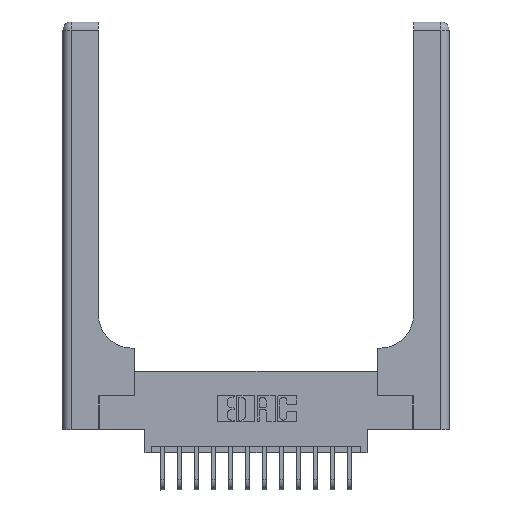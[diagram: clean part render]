
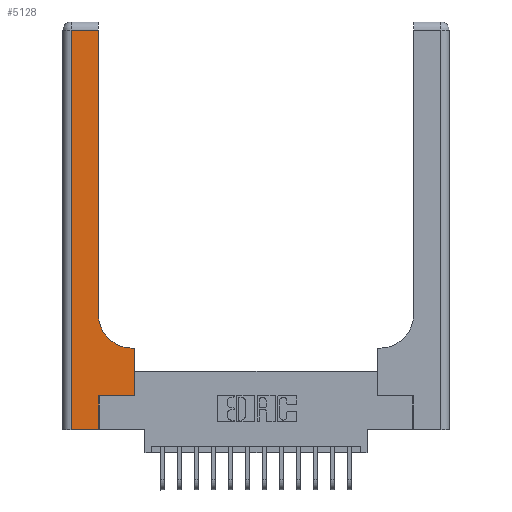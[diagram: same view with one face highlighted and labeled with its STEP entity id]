
A CAD part, top view. The second image highlights one B-rep face of the part: STEP entity #5128.
In plain terms, the highlighted planar face has unit normal (0, 0, 1).
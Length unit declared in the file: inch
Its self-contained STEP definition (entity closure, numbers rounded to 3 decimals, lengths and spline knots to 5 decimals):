
#183 = VERTEX_POINT ( 'NONE', #13406 ) ;
#333 = CARTESIAN_POINT ( 'NONE',  ( 0.06, 0., 0.37 ) ) ;
#395 = LINE ( 'NONE', #5743, #4962 ) ;
#425 = ORIENTED_EDGE ( 'NONE', *, *, #15638, .T. ) ;
#802 = VERTEX_POINT ( 'NONE', #10379 ) ;
#989 = ORIENTED_EDGE ( 'NONE', *, *, #3616, .T. ) ;
#1269 = EDGE_CURVE ( 'NONE', #12858, #1861, #12002, .T. ) ;
#1292 = DIRECTION ( 'NONE',  ( -1., 0., 0. ) ) ;
#1320 = DIRECTION ( 'NONE',  ( 1., 0., 0. ) ) ;
#1595 = LINE ( 'NONE', #17290, #9829 ) ;
#1654 = ORIENTED_EDGE ( 'NONE', *, *, #13908, .T. ) ;
#1861 = VERTEX_POINT ( 'NONE', #13651 ) ;
#2152 = VERTEX_POINT ( 'NONE', #13627 ) ;
#2262 = EDGE_CURVE ( 'NONE', #183, #13334, #3917, .T. ) ;
#2563 = EDGE_CURVE ( 'NONE', #5807, #802, #9725, .T. ) ;
#2675 = CARTESIAN_POINT ( 'NONE',  ( 0., 2.94, 0.37 ) ) ;
#2682 = CARTESIAN_POINT ( 'NONE',  ( 0.265, 0.25, 0.37 ) ) ;
#2789 = DIRECTION ( 'NONE',  ( -1., 0., 0. ) ) ;
#3233 = ORIENTED_EDGE ( 'NONE', *, *, #17201, .T. ) ;
#3318 = DIRECTION ( 'NONE',  ( 0., -1., 0. ) ) ;
#3373 = EDGE_CURVE ( 'NONE', #802, #12858, #7390, .T. ) ;
#3417 = CARTESIAN_POINT ( 'NONE',  ( 0.51, 0.85, 0.37 ) ) ;
#3509 = VERTEX_POINT ( 'NONE', #16862 ) ;
#3616 = EDGE_CURVE ( 'NONE', #1861, #3509, #1595, .T. ) ;
#3917 = CIRCLE ( 'NONE', #12902, 0.25 ) ;
#4319 = VECTOR ( 'NONE', #3318, 39.37008 ) ;
#4962 = VECTOR ( 'NONE', #12499, 39.37008 ) ;
#5128 = ADVANCED_FACE ( 'NONE', ( #17272 ), #9367, .F. ) ;
#5510 = CARTESIAN_POINT ( 'NONE',  ( 0.265, 0.25, 0.37 ) ) ;
#5743 = CARTESIAN_POINT ( 'NONE',  ( 0.26, 0.6, 0.37 ) ) ;
#5748 = ORIENTED_EDGE ( 'NONE', *, *, #7207, .T. ) ;
#5807 = VERTEX_POINT ( 'NONE', #333 ) ;
#6275 = VECTOR ( 'NONE', #13672, 39.37008 ) ;
#6960 = LINE ( 'NONE', #2675, #16210 ) ;
#7075 = CARTESIAN_POINT ( 'NONE',  ( 0.06, 3., 0.37 ) ) ;
#7207 = EDGE_CURVE ( 'NONE', #13334, #12428, #16456, .T. ) ;
#7390 = LINE ( 'NONE', #15204, #15443 ) ;
#7636 = DIRECTION ( 'NONE',  ( 0., 0., -1. ) ) ;
#8068 = ORIENTED_EDGE ( 'NONE', *, *, #1269, .T. ) ;
#8436 = CARTESIAN_POINT ( 'NONE',  ( 0.26, 0.85, 0.37 ) ) ;
#8875 = DIRECTION ( 'NONE',  ( 1., 0., 0. ) ) ;
#9319 = VECTOR ( 'NONE', #11112, 39.37008 ) ;
#9367 = PLANE ( 'NONE',  #9828 ) ;
#9725 = LINE ( 'NONE', #12353, #6275 ) ;
#9767 = DIRECTION ( 'NONE',  ( 0., 1., 0. ) ) ;
#9828 = AXIS2_PLACEMENT_3D ( 'NONE', #16124, #12092, #2789 ) ;
#9829 = VECTOR ( 'NONE', #15964, 39.37008 ) ;
#9986 = ORIENTED_EDGE ( 'NONE', *, *, #3373, .T. ) ;
#10379 = CARTESIAN_POINT ( 'NONE',  ( 0.265, 0., 0.37 ) ) ;
#11112 = DIRECTION ( 'NONE',  ( 0., 1., 0. ) ) ;
#12002 = LINE ( 'NONE', #5510, #16115 ) ;
#12092 = DIRECTION ( 'NONE',  ( 0., 0., -1. ) ) ;
#12353 = CARTESIAN_POINT ( 'NONE',  ( 0., 0., 0.37 ) ) ;
#12428 = VERTEX_POINT ( 'NONE', #17181 ) ;
#12499 = DIRECTION ( 'NONE',  ( -1., 0., 0. ) ) ;
#12858 = VERTEX_POINT ( 'NONE', #2682 ) ;
#12902 = AXIS2_PLACEMENT_3D ( 'NONE', #3417, #7636, #8875 ) ;
#13186 = EDGE_LOOP ( 'NONE', ( #5748, #425, #3233, #14828, #9986, #8068, #989, #1654, #17090 ) ) ;
#13334 = VERTEX_POINT ( 'NONE', #8436 ) ;
#13406 = CARTESIAN_POINT ( 'NONE',  ( 0.51, 0.6, 0.37 ) ) ;
#13627 = CARTESIAN_POINT ( 'NONE',  ( 0.06, 2.94, 0.37 ) ) ;
#13651 = CARTESIAN_POINT ( 'NONE',  ( 0.528, 0.25, 0.37 ) ) ;
#13672 = DIRECTION ( 'NONE',  ( 1., 0., 0. ) ) ;
#13853 = LINE ( 'NONE', #7075, #4319 ) ;
#13908 = EDGE_CURVE ( 'NONE', #3509, #183, #395, .T. ) ;
#14828 = ORIENTED_EDGE ( 'NONE', *, *, #2563, .T. ) ;
#15204 = CARTESIAN_POINT ( 'NONE',  ( 0.265, 0., 0.37 ) ) ;
#15443 = VECTOR ( 'NONE', #9767, 39.37008 ) ;
#15638 = EDGE_CURVE ( 'NONE', #12428, #2152, #6960, .T. ) ;
#15964 = DIRECTION ( 'NONE',  ( 0., 1., 0. ) ) ;
#16115 = VECTOR ( 'NONE', #1320, 39.37008 ) ;
#16124 = CARTESIAN_POINT ( 'NONE',  ( 0., 3., 0.37 ) ) ;
#16210 = VECTOR ( 'NONE', #1292, 39.37008 ) ;
#16366 = CARTESIAN_POINT ( 'NONE',  ( 0.26, 3., 0.37 ) ) ;
#16456 = LINE ( 'NONE', #16366, #9319 ) ;
#16862 = CARTESIAN_POINT ( 'NONE',  ( 0.528, 0.6, 0.37 ) ) ;
#17090 = ORIENTED_EDGE ( 'NONE', *, *, #2262, .T. ) ;
#17181 = CARTESIAN_POINT ( 'NONE',  ( 0.26, 2.94, 0.37 ) ) ;
#17201 = EDGE_CURVE ( 'NONE', #2152, #5807, #13853, .T. ) ;
#17272 = FACE_OUTER_BOUND ( 'NONE', #13186, .T. ) ;
#17290 = CARTESIAN_POINT ( 'NONE',  ( 0.528, 0.25, 0.37 ) ) ;
